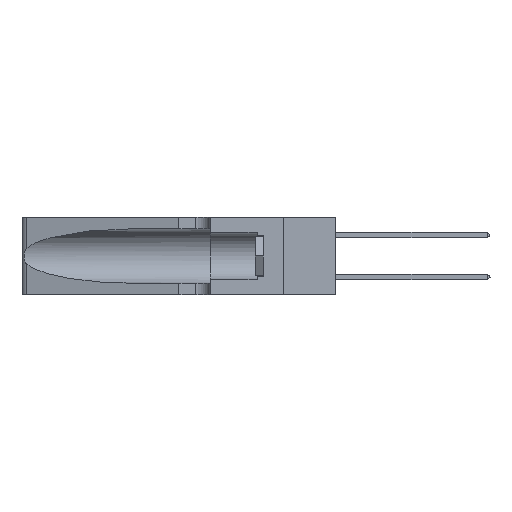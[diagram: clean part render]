
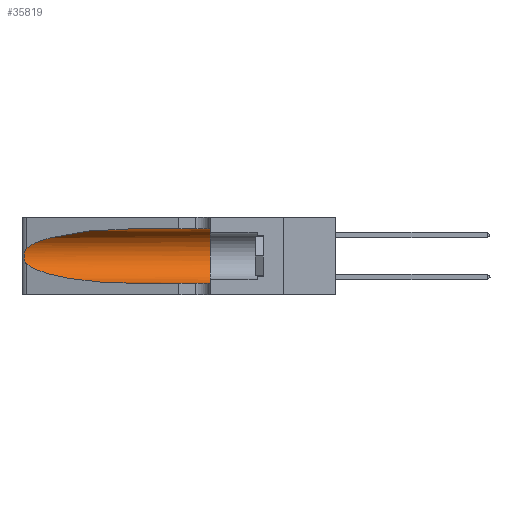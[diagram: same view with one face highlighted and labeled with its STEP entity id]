
A CAD part, left-side view. The second image highlights one B-rep face of the part: STEP entity #35819.
In plain terms, the highlighted cylindrical face has radius 3.308 mm (diameter 6.617 mm), a partial arc.
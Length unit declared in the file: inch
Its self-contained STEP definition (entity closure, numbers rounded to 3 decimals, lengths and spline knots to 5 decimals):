
#341 = LINE ( 'NONE', #38563, #25759 ) ;
#581 = CARTESIAN_POINT ( 'NONE',  ( 0.1305, 0.35, 0.05475 ) ) ;
#1543 = EDGE_CURVE ( 'NONE', #21874, #27685, #32252, .T. ) ;
#1752 = VERTEX_POINT ( 'NONE', #7758 ) ;
#2702 = AXIS2_PLACEMENT_3D ( 'NONE', #14891, #8512, #36546 ) ;
#3582 = VERTEX_POINT ( 'NONE', #21339 ) ;
#3739 = CARTESIAN_POINT ( 'NONE',  ( 0.1305, 1.61858, 0.31525 ) ) ;
#5061 = CARTESIAN_POINT ( 'NONE',  ( 0.2373, 1.15595, 0.08982 ) ) ;
#6603 = DIRECTION ( 'NONE',  ( 0., 0., 1. ) ) ;
#6888 = CARTESIAN_POINT ( 'NONE',  ( 0.25854, 1.2359, 0.20912 ) ) ;
#6906 = DIRECTION ( 'NONE',  ( 0., -1., 0. ) ) ;
#7089 = CARTESIAN_POINT ( 'NONE',  ( 0.25487, 1.22718, 0.14631 ) ) ;
#7758 = CARTESIAN_POINT ( 'NONE',  ( 0.25487, 1.22718, 0.22369 ) ) ;
#8205 = CARTESIAN_POINT ( 'NONE',  ( 0.18966, 0.96281, 0.05475 ) ) ;
#8445 = B_SPLINE_CURVE_WITH_KNOTS ( 'NONE', 3,
 ( #16012, #25872, #31603, #29043, #6888, #10322, #37849, #13050, #28499, #22423, #32139, #35231, #28625, #13198 ),
 .UNSPECIFIED., .F., .F.,
 ( 4, 2, 2, 2, 2, 2, 4 ),
 ( 0., 0.00027, 0.00053, 0.00107, 0.0016, 0.00187, 0.00214 ),
 .UNSPECIFIED. ) ;
#8512 = DIRECTION ( 'NONE',  ( 0., -1., 0. ) ) ;
#9412 = CARTESIAN_POINT ( 'NONE',  ( 0.25487, 1.22718, 0.22369 ) ) ;
#9900 = EDGE_CURVE ( 'NONE', #27685, #31348, #25293, .T. ) ;
#10322 = CARTESIAN_POINT ( 'NONE',  ( 0.26018, 1.23835, 0.19895 ) ) ;
#10754 = CARTESIAN_POINT ( 'NONE',  ( 0.1305, 0.35, 0.185 ) ) ;
#11335 = CARTESIAN_POINT ( 'NONE',  ( 0.1305, 0.72297, 0.05475 ) ) ;
#12135 = CARTESIAN_POINT ( 'NONE',  ( 0.1305, 0.72297, 0.31525 ) ) ;
#12398 = CARTESIAN_POINT ( 'NONE',  ( 0.1305, 0.72297, 0.31525 ) ) ;
#13050 = CARTESIAN_POINT ( 'NONE',  ( 0.26075, 1.23896, 0.178 ) ) ;
#13198 = CARTESIAN_POINT ( 'NONE',  ( 0.25487, 1.22718, 0.14631 ) ) ;
#13208 = EDGE_CURVE ( 'NONE', #3582, #31348, #341, .T. ) ;
#13768 = ORIENTED_EDGE ( 'NONE', *, *, #24300, .T. ) ;
#13894 = DIRECTION ( 'NONE',  ( 0., 1., 0. ) ) ;
#14891 = CARTESIAN_POINT ( 'NONE',  ( 0.1305, 1.61858, 0.185 ) ) ;
#15591 = ORIENTED_EDGE ( 'NONE', *, *, #34829, .T. ) ;
#16012 = CARTESIAN_POINT ( 'NONE',  ( 0.25487, 1.22718, 0.22369 ) ) ;
#18279 = ORIENTED_EDGE ( 'NONE', *, *, #1543, .F. ) ;
#19601 = DIRECTION ( 'NONE',  ( 0., -1., 0. ) ) ;
#21339 = CARTESIAN_POINT ( 'NONE',  ( 0.1305, 0.72297, 0.05475 ) ) ;
#21874 = VERTEX_POINT ( 'NONE', #12398 ) ;
#22423 = CARTESIAN_POINT ( 'NONE',  ( 0.25856, 1.23593, 0.16098 ) ) ;
#23544 = AXIS2_PLACEMENT_3D ( 'NONE', #10754, #13894, #6603 ) ;
#23663 = CARTESIAN_POINT ( 'NONE',  ( 0.1305, 0.35, 0.31525 ) ) ;
#24183 =( BOUNDED_CURVE ( )  B_SPLINE_CURVE ( 3, ( #27193, #5061, #8205, #11335 ),
 .UNSPECIFIED., .F., .F. ) 
 B_SPLINE_CURVE_WITH_KNOTS ( ( 4, 4 ),
 ( 3.44316, 4.71239 ),
 .UNSPECIFIED. ) 
 CURVE ( )  GEOMETRIC_REPRESENTATION_ITEM ( )  RATIONAL_B_SPLINE_CURVE ( ( 1., 0.87, 0.87, 1. ) ) 
 REPRESENTATION_ITEM ( '' )  );
#24300 = EDGE_CURVE ( 'NONE', #26260, #3582, #24183, .T. ) ;
#24696 = CARTESIAN_POINT ( 'NONE',  ( 0.2373, 1.15595, 0.28018 ) ) ;
#25293 = CIRCLE ( 'NONE', #23544, 0.13025 ) ;
#25359 = EDGE_CURVE ( 'NONE', #21874, #1752, #38642, .T. ) ;
#25759 = VECTOR ( 'NONE', #19601, 39.37008 ) ;
#25872 = CARTESIAN_POINT ( 'NONE',  ( 0.25555, 1.22994, 0.2215 ) ) ;
#26260 = VERTEX_POINT ( 'NONE', #7089 ) ;
#26501 = ORIENTED_EDGE ( 'NONE', *, *, #9900, .F. ) ;
#27193 = CARTESIAN_POINT ( 'NONE',  ( 0.25487, 1.22718, 0.14631 ) ) ;
#27685 = VERTEX_POINT ( 'NONE', #23663 ) ;
#28499 = CARTESIAN_POINT ( 'NONE',  ( 0.26017, 1.23833, 0.17102 ) ) ;
#28625 = CARTESIAN_POINT ( 'NONE',  ( 0.25555, 1.22993, 0.14849 ) ) ;
#28867 = VECTOR ( 'NONE', #6906, 39.37008 ) ;
#29043 = CARTESIAN_POINT ( 'NONE',  ( 0.25787, 1.23484, 0.2124 ) ) ;
#31348 = VERTEX_POINT ( 'NONE', #581 ) ;
#31603 = CARTESIAN_POINT ( 'NONE',  ( 0.25639, 1.23184, 0.21858 ) ) ;
#31706 = CYLINDRICAL_SURFACE ( 'NONE', #2702, 0.13025 ) ;
#32139 = CARTESIAN_POINT ( 'NONE',  ( 0.25789, 1.23486, 0.15765 ) ) ;
#32252 = LINE ( 'NONE', #3739, #28867 ) ;
#32714 = FACE_OUTER_BOUND ( 'NONE', #33644, .T. ) ;
#33644 = EDGE_LOOP ( 'NONE', ( #34253, #15591, #13768, #34235, #26501, #18279 ) ) ;
#34235 = ORIENTED_EDGE ( 'NONE', *, *, #13208, .T. ) ;
#34253 = ORIENTED_EDGE ( 'NONE', *, *, #25359, .T. ) ;
#34829 = EDGE_CURVE ( 'NONE', #1752, #26260, #8445, .T. ) ;
#35231 = CARTESIAN_POINT ( 'NONE',  ( 0.25639, 1.23186, 0.15144 ) ) ;
#35819 = ADVANCED_FACE ( 'NONE', ( #32714 ), #31706, .F. ) ;
#36546 = DIRECTION ( 'NONE',  ( 0., 0., -1. ) ) ;
#36938 = CARTESIAN_POINT ( 'NONE',  ( 0.18966, 0.96281, 0.31525 ) ) ;
#37849 = CARTESIAN_POINT ( 'NONE',  ( 0.26075, 1.23896, 0.19203 ) ) ;
#38563 = CARTESIAN_POINT ( 'NONE',  ( 0.1305, 1.61858, 0.05475 ) ) ;
#38642 =( BOUNDED_CURVE ( )  B_SPLINE_CURVE ( 3, ( #12135, #36938, #24696, #9412 ),
 .UNSPECIFIED., .F., .F. ) 
 B_SPLINE_CURVE_WITH_KNOTS ( ( 4, 4 ),
 ( 1.5708, 2.84003 ),
 .UNSPECIFIED. ) 
 CURVE ( )  GEOMETRIC_REPRESENTATION_ITEM ( )  RATIONAL_B_SPLINE_CURVE ( ( 1., 0.87, 0.87, 1. ) ) 
 REPRESENTATION_ITEM ( '' )  );
